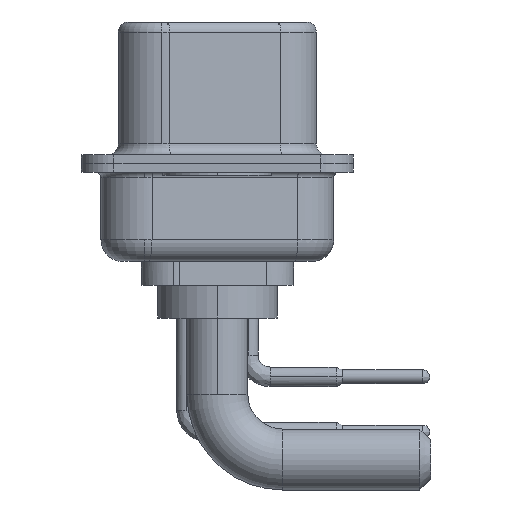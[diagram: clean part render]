
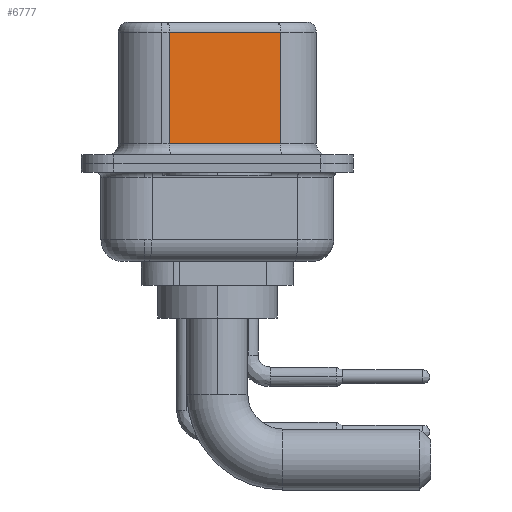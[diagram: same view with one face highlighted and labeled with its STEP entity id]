
A CAD part, left-side view. The second image highlights one B-rep face of the part: STEP entity #6777.
In plain terms, the highlighted planar face has unit normal (-0.985, -0.174, 0).
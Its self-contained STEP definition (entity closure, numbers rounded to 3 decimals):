
#1044 = VECTOR ( 'NONE', #21315, 1000. ) ;
#2616 = VECTOR ( 'NONE', #25204, 1000. ) ;
#3249 = CARTESIAN_POINT ( 'NONE',  ( 3.68, 2.203, 0.9 ) ) ;
#3308 = LINE ( 'NONE', #21716, #1044 ) ;
#3609 = ORIENTED_EDGE ( 'NONE', *, *, #15097, .T. ) ;
#5492 = ORIENTED_EDGE ( 'NONE', *, *, #26130, .T. ) ;
#5533 = VERTEX_POINT ( 'NONE', #7182 ) ;
#6281 = CARTESIAN_POINT ( 'NONE',  ( 4.58, -2.897, 6.02 ) ) ;
#6777 = ADVANCED_FACE ( 'NONE', ( #20236 ), #7492, .F. ) ;
#7182 = CARTESIAN_POINT ( 'NONE',  ( 4.58, -2.897, 0.9 ) ) ;
#7492 = PLANE ( 'NONE',  #17684 ) ;
#8392 = LINE ( 'NONE', #18984, #2616 ) ;
#9070 = VERTEX_POINT ( 'NONE', #3249 ) ;
#9846 = ORIENTED_EDGE ( 'NONE', *, *, #21293, .F. ) ;
#10124 = LINE ( 'NONE', #24514, #18892 ) ;
#10308 = EDGE_LOOP ( 'NONE', ( #9846, #5492, #3609, #22393 ) ) ;
#10915 = DIRECTION ( 'NONE',  ( 0., 0., -1. ) ) ;
#11821 = DIRECTION ( 'NONE',  ( 0.985, 0.174, 0. ) ) ;
#12319 = VECTOR ( 'NONE', #10915, 1000. ) ;
#13898 = VERTEX_POINT ( 'NONE', #16732 ) ;
#15097 = EDGE_CURVE ( 'NONE', #13898, #9070, #26662, .T. ) ;
#15422 = CARTESIAN_POINT ( 'NONE',  ( 3.68, 2.203, 6.52 ) ) ;
#16166 = CARTESIAN_POINT ( 'NONE',  ( 4.58, -2.897, 6.52 ) ) ;
#16732 = CARTESIAN_POINT ( 'NONE',  ( 3.68, 2.203, 6.02 ) ) ;
#17183 = VERTEX_POINT ( 'NONE', #6281 ) ;
#17684 = AXIS2_PLACEMENT_3D ( 'NONE', #16166, #11821, #22384 ) ;
#17997 = EDGE_CURVE ( 'NONE', #9070, #5533, #10124, .T. ) ;
#18892 = VECTOR ( 'NONE', #26530, 1000. ) ;
#18984 = CARTESIAN_POINT ( 'NONE',  ( 4.58, -2.897, 6.52 ) ) ;
#20236 = FACE_OUTER_BOUND ( 'NONE', #10308, .T. ) ;
#21293 = EDGE_CURVE ( 'NONE', #17183, #5533, #8392, .T. ) ;
#21315 = DIRECTION ( 'NONE',  ( -0.174, 0.985, 0. ) ) ;
#21716 = CARTESIAN_POINT ( 'NONE',  ( 4.58, -2.897, 6.02 ) ) ;
#22384 = DIRECTION ( 'NONE',  ( -0.174, 0.985, 0. ) ) ;
#22393 = ORIENTED_EDGE ( 'NONE', *, *, #17997, .T. ) ;
#24514 = CARTESIAN_POINT ( 'NONE',  ( 4.58, -2.897, 0.9 ) ) ;
#25204 = DIRECTION ( 'NONE',  ( 0., 0., -1. ) ) ;
#26130 = EDGE_CURVE ( 'NONE', #17183, #13898, #3308, .T. ) ;
#26530 = DIRECTION ( 'NONE',  ( 0.174, -0.985, 0. ) ) ;
#26662 = LINE ( 'NONE', #15422, #12319 ) ;
